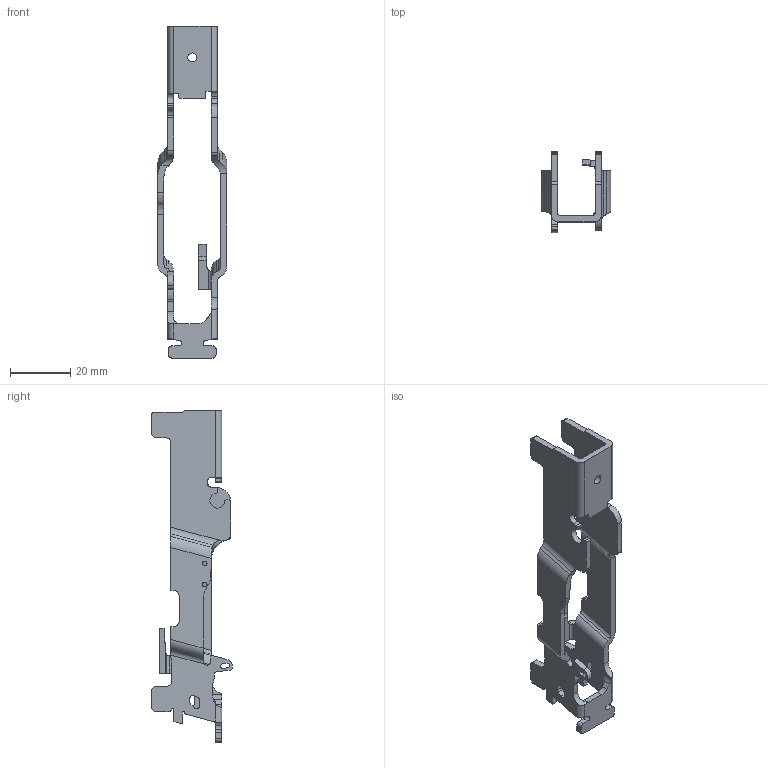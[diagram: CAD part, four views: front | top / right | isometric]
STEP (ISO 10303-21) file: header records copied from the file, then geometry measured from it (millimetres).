
FILE_DESCRIPTION(/* description */ (''),/* implementation_level */ '2;1');
FILE_NAME(/* name */ '320 FCU Bent Blank.step',/* time_stamp */ '2021-04-10T07:32:26-04:00',/* author */ (''),/* organization */ (''),/* preprocessor_version */ 'ST-DEVELOPER v18.1',/* originating_system */ 'Autodesk Translation Framework v10.6.0.1341',/* authorisation */ '');
FILE_SCHEMA (('AUTOMOTIVE_DESIGN { 1 0 10303 214 3 1 1 }'));
Length unit declared in the file: millimetre
Products named in the file (1): 320 FCU no holes
Bounding box: 23.15 x 26.83 x 110.25 mm (x, y, z)
Volume: 7583.6 mm3; surface area: 8934.7 mm2
Topology: 1 solids, 1 shells, 226 faces, 668 edges, 444 vertices
Faces by surface type: plane 120, cylinder 104, torus 2
Full cylindrical faces by diameter (mm): 1.6 x2, 3 x1
Entity records: 7776 total; most frequent: CARTESIAN_POINT 1515, ORIENTED_EDGE 1336, DIRECTION 1311, EDGE_CURVE 668, VERTEX_POINT 444, AXIS2_PLACEMENT_3D 438, LINE 435, VECTOR 435
